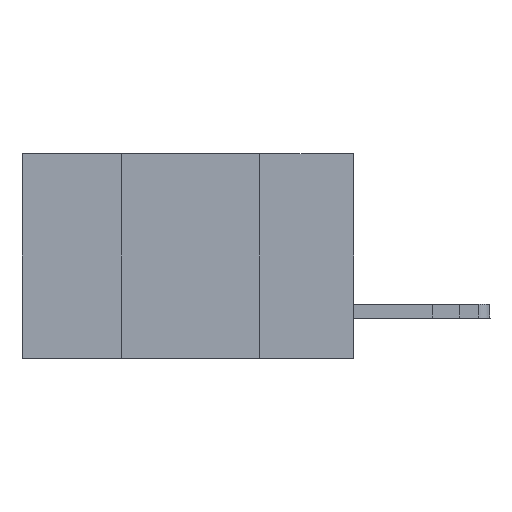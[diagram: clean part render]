
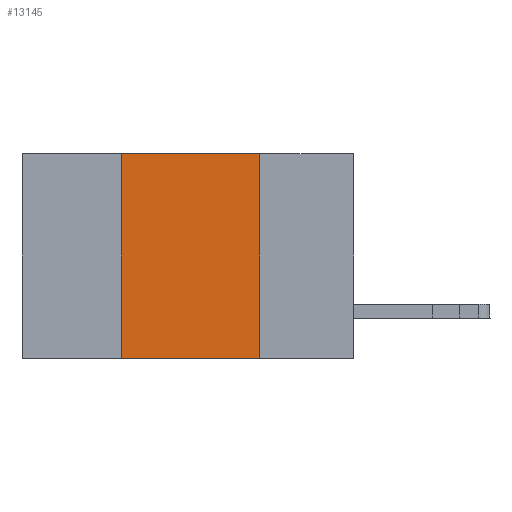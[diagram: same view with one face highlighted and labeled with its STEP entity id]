
A CAD part, left-side view. The second image highlights one B-rep face of the part: STEP entity #13145.
In plain terms, the highlighted planar face has unit normal (-1, 0, 0).
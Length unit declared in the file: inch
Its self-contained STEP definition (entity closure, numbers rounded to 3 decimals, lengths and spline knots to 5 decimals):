
#951 = CARTESIAN_POINT ( 'NONE',  ( 0., 0.42, 0. ) ) ;
#1135 = CARTESIAN_POINT ( 'NONE',  ( 0., 0.42, 0. ) ) ;
#2645 = DIRECTION ( 'NONE',  ( 0., -1., 0. ) ) ;
#3138 = ORIENTED_EDGE ( 'NONE', *, *, #21104, .F. ) ;
#4153 = LINE ( 'NONE', #12033, #19073 ) ;
#4494 = LINE ( 'NONE', #1135, #5086 ) ;
#4942 = PLANE ( 'NONE',  #12260 ) ;
#5086 = VECTOR ( 'NONE', #14308, 39.37008 ) ;
#6869 = DIRECTION ( 'NONE',  ( 0., 0., -1. ) ) ;
#6957 = CARTESIAN_POINT ( 'NONE',  ( 0., 0.17, -0.37 ) ) ;
#7038 = VERTEX_POINT ( 'NONE', #951 ) ;
#7309 = CARTESIAN_POINT ( 'NONE',  ( 0., 0.42, -0.37 ) ) ;
#7971 = EDGE_LOOP ( 'NONE', ( #9644, #14593, #3138, #16668 ) ) ;
#8666 = DIRECTION ( 'NONE',  ( 0., -1., 0. ) ) ;
#9052 = DIRECTION ( 'NONE',  ( 0., 0., -1. ) ) ;
#9644 = ORIENTED_EDGE ( 'NONE', *, *, #22328, .F. ) ;
#10427 = EDGE_CURVE ( 'NONE', #7038, #24144, #4153, .T. ) ;
#12033 = CARTESIAN_POINT ( 'NONE',  ( 0., 0.6, 0. ) ) ;
#12128 = VECTOR ( 'NONE', #9052, 39.37008 ) ;
#12260 = AXIS2_PLACEMENT_3D ( 'NONE', #21658, #18025, #6869 ) ;
#12345 = VECTOR ( 'NONE', #8666, 39.37008 ) ;
#13145 = ADVANCED_FACE ( 'NONE', ( #21555 ), #4942, .F. ) ;
#14308 = DIRECTION ( 'NONE',  ( 0., 0., 1. ) ) ;
#14593 = ORIENTED_EDGE ( 'NONE', *, *, #10427, .F. ) ;
#16057 = CARTESIAN_POINT ( 'NONE',  ( 0., 0.17, 0. ) ) ;
#16668 = ORIENTED_EDGE ( 'NONE', *, *, #19863, .T. ) ;
#17299 = LINE ( 'NONE', #21557, #12345 ) ;
#18025 = DIRECTION ( 'NONE',  ( 1., 0., 0. ) ) ;
#19073 = VECTOR ( 'NONE', #2645, 39.37008 ) ;
#19863 = EDGE_CURVE ( 'NONE', #20613, #21151, #17299, .T. ) ;
#20070 = CARTESIAN_POINT ( 'NONE',  ( 0., 0.17, 0. ) ) ;
#20613 = VERTEX_POINT ( 'NONE', #7309 ) ;
#21104 = EDGE_CURVE ( 'NONE', #20613, #7038, #4494, .T. ) ;
#21151 = VERTEX_POINT ( 'NONE', #6957 ) ;
#21401 = LINE ( 'NONE', #20070, #12128 ) ;
#21555 = FACE_OUTER_BOUND ( 'NONE', #7971, .T. ) ;
#21557 = CARTESIAN_POINT ( 'NONE',  ( 0., 0.6, -0.37 ) ) ;
#21658 = CARTESIAN_POINT ( 'NONE',  ( 0., 0.6, 0. ) ) ;
#22328 = EDGE_CURVE ( 'NONE', #24144, #21151, #21401, .T. ) ;
#24144 = VERTEX_POINT ( 'NONE', #16057 ) ;
